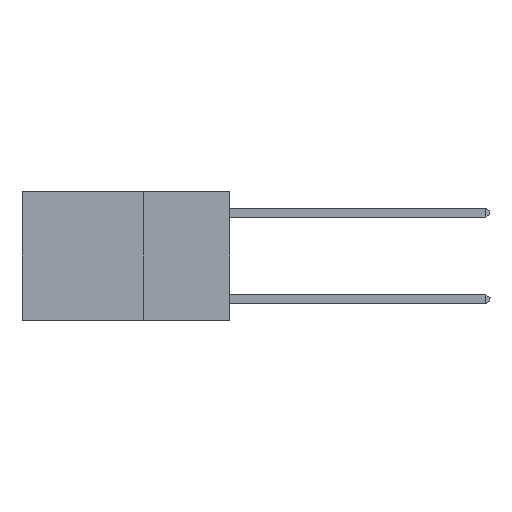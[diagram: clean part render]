
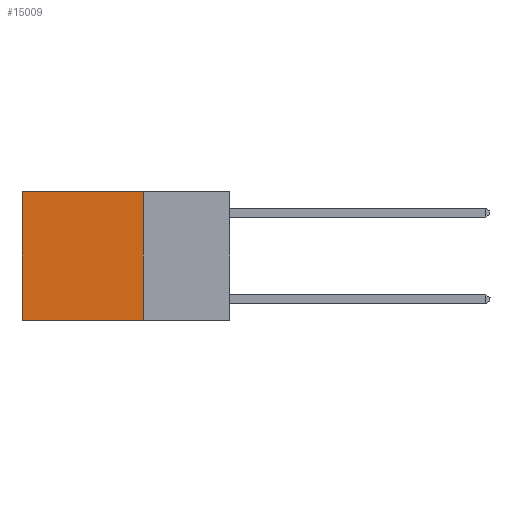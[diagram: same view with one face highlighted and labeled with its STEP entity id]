
A CAD part, left-side view. The second image highlights one B-rep face of the part: STEP entity #15009.
In plain terms, the highlighted planar face has unit normal (-1, 0, 0).
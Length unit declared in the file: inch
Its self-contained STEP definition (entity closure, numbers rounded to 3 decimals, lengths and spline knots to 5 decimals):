
#444 = CARTESIAN_POINT ( 'NONE',  ( 0.2625, 0.6, -0.37 ) ) ;
#581 = LINE ( 'NONE', #22455, #9229 ) ;
#1189 = VERTEX_POINT ( 'NONE', #444 ) ;
#1308 = EDGE_CURVE ( 'NONE', #22373, #20726, #15844, .T. ) ;
#2545 = VECTOR ( 'NONE', #4972, 39.37008 ) ;
#3587 = AXIS2_PLACEMENT_3D ( 'NONE', #6393, #20852, #10103 ) ;
#4491 = DIRECTION ( 'NONE',  ( 0., 0., -1. ) ) ;
#4518 = CARTESIAN_POINT ( 'NONE',  ( 0.2625, 0.6, 0. ) ) ;
#4972 = DIRECTION ( 'NONE',  ( 0., 1., 0. ) ) ;
#5222 = CARTESIAN_POINT ( 'NONE',  ( 0.2625, 0.6, 0. ) ) ;
#6167 = VECTOR ( 'NONE', #4491, 39.37008 ) ;
#6393 = CARTESIAN_POINT ( 'NONE',  ( 0.2625, 0.25, 0. ) ) ;
#6593 = EDGE_LOOP ( 'NONE', ( #17084, #16340, #15673, #20503 ) ) ;
#6894 = EDGE_CURVE ( 'NONE', #22373, #17830, #12850, .T. ) ;
#9229 = VECTOR ( 'NONE', #18873, 39.37008 ) ;
#10103 = DIRECTION ( 'NONE',  ( 0., 0., -1. ) ) ;
#11942 = CARTESIAN_POINT ( 'NONE',  ( 0.2625, 0.25, -0.37 ) ) ;
#12850 = LINE ( 'NONE', #15867, #2545 ) ;
#13530 = EDGE_CURVE ( 'NONE', #20726, #1189, #581, .T. ) ;
#15009 = ADVANCED_FACE ( 'NONE', ( #17626 ), #17263, .F. ) ;
#15673 = ORIENTED_EDGE ( 'NONE', *, *, #1308, .F. ) ;
#15844 = LINE ( 'NONE', #17203, #6167 ) ;
#15867 = CARTESIAN_POINT ( 'NONE',  ( 0.2625, 0.25, 0. ) ) ;
#16116 = DIRECTION ( 'NONE',  ( 0., 0., -1. ) ) ;
#16133 = EDGE_CURVE ( 'NONE', #17830, #1189, #16730, .T. ) ;
#16172 = VECTOR ( 'NONE', #16116, 39.37008 ) ;
#16340 = ORIENTED_EDGE ( 'NONE', *, *, #13530, .F. ) ;
#16730 = LINE ( 'NONE', #5222, #16172 ) ;
#17084 = ORIENTED_EDGE ( 'NONE', *, *, #16133, .T. ) ;
#17203 = CARTESIAN_POINT ( 'NONE',  ( 0.2625, 0.25, 0. ) ) ;
#17263 = PLANE ( 'NONE',  #3587 ) ;
#17626 = FACE_OUTER_BOUND ( 'NONE', #6593, .T. ) ;
#17830 = VERTEX_POINT ( 'NONE', #4518 ) ;
#18873 = DIRECTION ( 'NONE',  ( 0., 1., 0. ) ) ;
#19927 = CARTESIAN_POINT ( 'NONE',  ( 0.2625, 0.25, 0. ) ) ;
#20503 = ORIENTED_EDGE ( 'NONE', *, *, #6894, .T. ) ;
#20726 = VERTEX_POINT ( 'NONE', #11942 ) ;
#20852 = DIRECTION ( 'NONE',  ( 1., 0., 0. ) ) ;
#22373 = VERTEX_POINT ( 'NONE', #19927 ) ;
#22455 = CARTESIAN_POINT ( 'NONE',  ( 0.2625, 0.25, -0.37 ) ) ;
